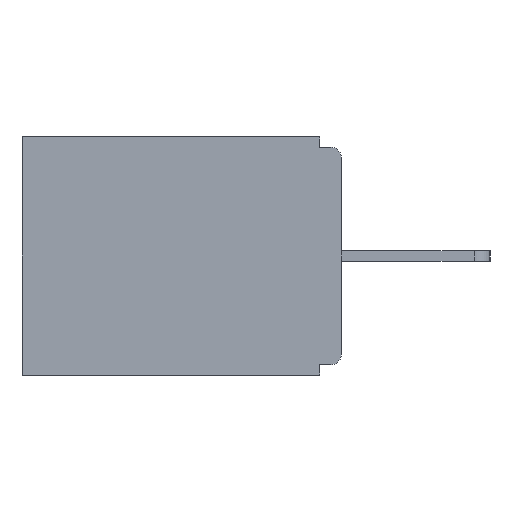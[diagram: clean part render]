
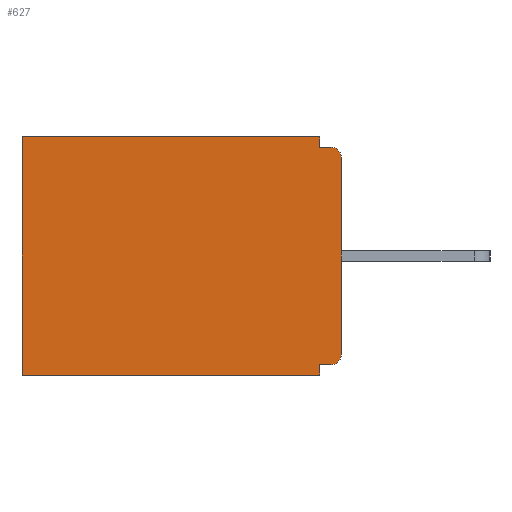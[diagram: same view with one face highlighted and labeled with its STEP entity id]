
A CAD part, left-side view. The second image highlights one B-rep face of the part: STEP entity #627.
In plain terms, the highlighted planar face has unit normal (-1, 0, 0).
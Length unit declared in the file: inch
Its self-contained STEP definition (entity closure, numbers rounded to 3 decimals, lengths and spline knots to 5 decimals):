
#39 = CARTESIAN_POINT ( 'NONE',  ( 0.298, 0., -0.313 ) ) ;
#102 = ORIENTED_EDGE ( 'NONE', *, *, #10883, .T. ) ;
#201 = CIRCLE ( 'NONE', #11126, 0.015 ) ;
#248 = VECTOR ( 'NONE', #12221, 39.37008 ) ;
#389 = EDGE_CURVE ( 'NONE', #3148, #4019, #8567, .T. ) ;
#529 = CARTESIAN_POINT ( 'NONE',  ( 0.298, 0.031, -0.343 ) ) ;
#627 = ADVANCED_FACE ( 'NONE', ( #13497 ), #3396, .F. ) ;
#681 = EDGE_CURVE ( 'NONE', #12133, #11183, #10634, .T. ) ;
#1035 = DIRECTION ( 'NONE',  ( 0., 0., -1. ) ) ;
#1825 = ORIENTED_EDGE ( 'NONE', *, *, #10726, .F. ) ;
#2323 = CARTESIAN_POINT ( 'NONE',  ( 0.298, 0., -0.03 ) ) ;
#2428 = CARTESIAN_POINT ( 'NONE',  ( 0.298, 0.015, -0.03 ) ) ;
#2684 = DIRECTION ( 'NONE',  ( 0., 0., -1. ) ) ;
#3091 = VERTEX_POINT ( 'NONE', #13465 ) ;
#3148 = VERTEX_POINT ( 'NONE', #2323 ) ;
#3306 = CARTESIAN_POINT ( 'NONE',  ( 0.298, 0.46, -0.343 ) ) ;
#3396 = PLANE ( 'NONE',  #16231 ) ;
#3465 = CARTESIAN_POINT ( 'NONE',  ( 0.298, 0., 0. ) ) ;
#3759 = CARTESIAN_POINT ( 'NONE',  ( 0.298, 0., 0. ) ) ;
#3822 = DIRECTION ( 'NONE',  ( -1., 0., 0. ) ) ;
#4019 = VERTEX_POINT ( 'NONE', #39 ) ;
#4447 = AXIS2_PLACEMENT_3D ( 'NONE', #2428, #3822, #13569 ) ;
#4986 = VECTOR ( 'NONE', #1035, 39.37008 ) ;
#5073 = CARTESIAN_POINT ( 'NONE',  ( 0.298, 0.015, -0.015 ) ) ;
#5205 = LINE ( 'NONE', #9366, #14586 ) ;
#5218 = DIRECTION ( 'NONE',  ( 0., 1., 0. ) ) ;
#5365 = VERTEX_POINT ( 'NONE', #13251 ) ;
#5515 = ORIENTED_EDGE ( 'NONE', *, *, #681, .F. ) ;
#5624 = CARTESIAN_POINT ( 'NONE',  ( 0.298, 0., -0.328 ) ) ;
#5702 = CARTESIAN_POINT ( 'NONE',  ( 0.298, 0.031, -0.015 ) ) ;
#6002 = DIRECTION ( 'NONE',  ( 1., 0., 0. ) ) ;
#6053 = VECTOR ( 'NONE', #8512, 39.37008 ) ;
#6122 = VERTEX_POINT ( 'NONE', #5073 ) ;
#6251 = LINE ( 'NONE', #6722, #14964 ) ;
#6555 = EDGE_CURVE ( 'NONE', #15345, #6122, #6251, .T. ) ;
#6722 = CARTESIAN_POINT ( 'NONE',  ( 0.298, 0., -0.015 ) ) ;
#7414 = EDGE_CURVE ( 'NONE', #17587, #4019, #201, .T. ) ;
#7595 = VECTOR ( 'NONE', #9186, 39.37008 ) ;
#7948 = ORIENTED_EDGE ( 'NONE', *, *, #6555, .F. ) ;
#8300 = ORIENTED_EDGE ( 'NONE', *, *, #12875, .T. ) ;
#8343 = VERTEX_POINT ( 'NONE', #16627 ) ;
#8512 = DIRECTION ( 'NONE',  ( 0., 1., 0. ) ) ;
#8567 = LINE ( 'NONE', #3759, #11406 ) ;
#9158 = DIRECTION ( 'NONE',  ( 0., 0., -1. ) ) ;
#9186 = DIRECTION ( 'NONE',  ( 0., 0., -1. ) ) ;
#9366 = CARTESIAN_POINT ( 'NONE',  ( 0.298, 0., 0. ) ) ;
#10387 = EDGE_CURVE ( 'NONE', #5365, #8343, #5205, .T. ) ;
#10634 = LINE ( 'NONE', #17751, #248 ) ;
#10726 = EDGE_CURVE ( 'NONE', #17587, #3091, #11052, .T. ) ;
#10883 = EDGE_CURVE ( 'NONE', #8343, #11183, #16087, .T. ) ;
#11019 = ORIENTED_EDGE ( 'NONE', *, *, #13441, .F. ) ;
#11052 = LINE ( 'NONE', #5624, #6053 ) ;
#11082 = CARTESIAN_POINT ( 'NONE',  ( 0.298, 0.015, -0.328 ) ) ;
#11126 = AXIS2_PLACEMENT_3D ( 'NONE', #12013, #16201, #9158 ) ;
#11183 = VERTEX_POINT ( 'NONE', #3306 ) ;
#11360 = ORIENTED_EDGE ( 'NONE', *, *, #12412, .F. ) ;
#11406 = VECTOR ( 'NONE', #2684, 39.37008 ) ;
#12013 = CARTESIAN_POINT ( 'NONE',  ( 0.298, 0.015, -0.313 ) ) ;
#12133 = VERTEX_POINT ( 'NONE', #529 ) ;
#12221 = DIRECTION ( 'NONE',  ( 0., 1., 0. ) ) ;
#12240 = DIRECTION ( 'NONE',  ( 0., 0., -1. ) ) ;
#12302 = CARTESIAN_POINT ( 'NONE',  ( 0.298, 0.031, -0.343 ) ) ;
#12412 = EDGE_CURVE ( 'NONE', #5365, #15345, #14716, .T. ) ;
#12875 = EDGE_CURVE ( 'NONE', #3148, #6122, #14060, .T. ) ;
#13251 = CARTESIAN_POINT ( 'NONE',  ( 0.298, 0.031, 0. ) ) ;
#13441 = EDGE_CURVE ( 'NONE', #3091, #12133, #16971, .T. ) ;
#13465 = CARTESIAN_POINT ( 'NONE',  ( 0.298, 0.031, -0.328 ) ) ;
#13495 = CARTESIAN_POINT ( 'NONE',  ( 0.298, 0.031, -0.343 ) ) ;
#13497 = FACE_OUTER_BOUND ( 'NONE', #15352, .T. ) ;
#13569 = DIRECTION ( 'NONE',  ( 0., 0., -1. ) ) ;
#14060 = CIRCLE ( 'NONE', #4447, 0.015 ) ;
#14586 = VECTOR ( 'NONE', #5218, 39.37008 ) ;
#14614 = DIRECTION ( 'NONE',  ( 0., 0., -1. ) ) ;
#14716 = LINE ( 'NONE', #12302, #15132 ) ;
#14964 = VECTOR ( 'NONE', #16443, 39.37008 ) ;
#15132 = VECTOR ( 'NONE', #12240, 39.37008 ) ;
#15345 = VERTEX_POINT ( 'NONE', #5702 ) ;
#15352 = EDGE_LOOP ( 'NONE', ( #8300, #7948, #11360, #16042, #102, #5515, #11019, #1825, #15948, #16396 ) ) ;
#15948 = ORIENTED_EDGE ( 'NONE', *, *, #7414, .T. ) ;
#16042 = ORIENTED_EDGE ( 'NONE', *, *, #10387, .T. ) ;
#16087 = LINE ( 'NONE', #17694, #7595 ) ;
#16201 = DIRECTION ( 'NONE',  ( -1., 0., 0. ) ) ;
#16231 = AXIS2_PLACEMENT_3D ( 'NONE', #3465, #6002, #14614 ) ;
#16396 = ORIENTED_EDGE ( 'NONE', *, *, #389, .F. ) ;
#16443 = DIRECTION ( 'NONE',  ( 0., -1., 0. ) ) ;
#16627 = CARTESIAN_POINT ( 'NONE',  ( 0.298, 0.46, 0. ) ) ;
#16971 = LINE ( 'NONE', #13495, #4986 ) ;
#17587 = VERTEX_POINT ( 'NONE', #11082 ) ;
#17694 = CARTESIAN_POINT ( 'NONE',  ( 0.298, 0.46, 0. ) ) ;
#17751 = CARTESIAN_POINT ( 'NONE',  ( 0.298, 0., -0.343 ) ) ;
